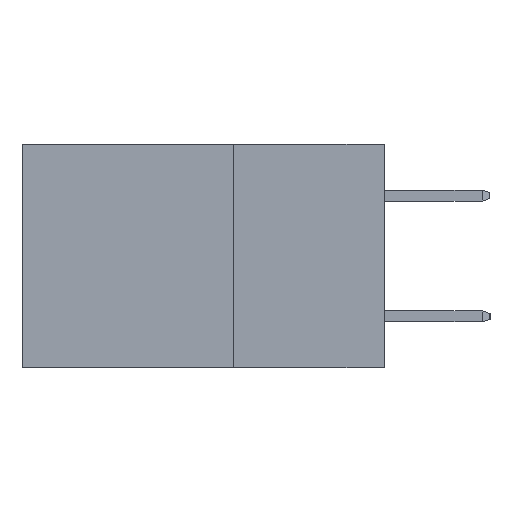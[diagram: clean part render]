
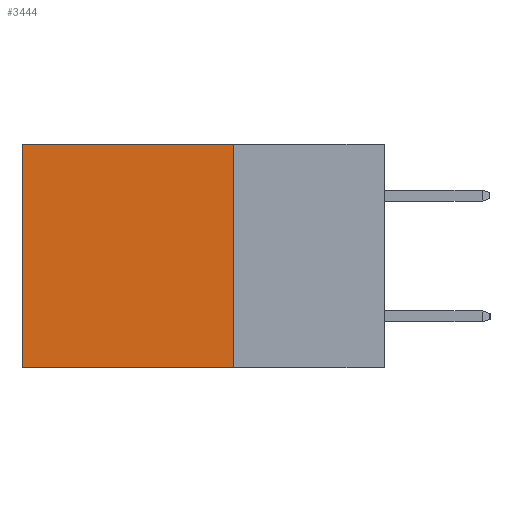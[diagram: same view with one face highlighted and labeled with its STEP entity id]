
A CAD part, left-side view. The second image highlights one B-rep face of the part: STEP entity #3444.
In plain terms, the highlighted planar face has unit normal (-1, 0, 0).
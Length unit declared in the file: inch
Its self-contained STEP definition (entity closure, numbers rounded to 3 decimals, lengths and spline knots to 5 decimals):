
#657 = CARTESIAN_POINT ( 'NONE',  ( 0.2615, 0.25, -0.37 ) ) ;
#1102 = ORIENTED_EDGE ( 'NONE', *, *, #1805, .T. ) ;
#1210 = EDGE_CURVE ( 'NONE', #1348, #4606, #9111, .T. ) ;
#1348 = VERTEX_POINT ( 'NONE', #11671 ) ;
#1699 = EDGE_CURVE ( 'NONE', #2932, #10370, #4565, .T. ) ;
#1805 = EDGE_CURVE ( 'NONE', #2932, #1348, #9880, .T. ) ;
#2069 = EDGE_CURVE ( 'NONE', #10370, #4606, #5583, .T. ) ;
#2316 = DIRECTION ( 'NONE',  ( 0., 0., -1. ) ) ;
#2762 = CARTESIAN_POINT ( 'NONE',  ( 0.2615, 0.25, -0.37 ) ) ;
#2932 = VERTEX_POINT ( 'NONE', #6329 ) ;
#3020 = ORIENTED_EDGE ( 'NONE', *, *, #2069, .F. ) ;
#3444 = ADVANCED_FACE ( 'NONE', ( #4428 ), #8945, .F. ) ;
#3583 = CARTESIAN_POINT ( 'NONE',  ( 0.2615, 0.25, -0.37 ) ) ;
#4061 = ORIENTED_EDGE ( 'NONE', *, *, #1210, .T. ) ;
#4428 = FACE_OUTER_BOUND ( 'NONE', #6059, .T. ) ;
#4563 = DIRECTION ( 'NONE',  ( 0., 0., -1. ) ) ;
#4565 = LINE ( 'NONE', #6421, #8715 ) ;
#4606 = VERTEX_POINT ( 'NONE', #6976 ) ;
#4660 = DIRECTION ( 'NONE',  ( 0., 1., 0. ) ) ;
#4981 = ORIENTED_EDGE ( 'NONE', *, *, #1699, .F. ) ;
#4996 = VECTOR ( 'NONE', #7368, 39.37008 ) ;
#5430 = CARTESIAN_POINT ( 'NONE',  ( 0.2615, 0.6, -0.37 ) ) ;
#5583 = LINE ( 'NONE', #3583, #9651 ) ;
#6059 = EDGE_LOOP ( 'NONE', ( #4061, #3020, #4981, #1102 ) ) ;
#6329 = CARTESIAN_POINT ( 'NONE',  ( 0.2615, 0.25, 0. ) ) ;
#6421 = CARTESIAN_POINT ( 'NONE',  ( 0.2615, 0.25, -0.37 ) ) ;
#6976 = CARTESIAN_POINT ( 'NONE',  ( 0.2615, 0.6, -0.37 ) ) ;
#7368 = DIRECTION ( 'NONE',  ( 0., 1., 0. ) ) ;
#8715 = VECTOR ( 'NONE', #10848, 39.37008 ) ;
#8945 = PLANE ( 'NONE',  #9903 ) ;
#9006 = CARTESIAN_POINT ( 'NONE',  ( 0.2615, 0.25, 0. ) ) ;
#9111 = LINE ( 'NONE', #5430, #10800 ) ;
#9651 = VECTOR ( 'NONE', #4660, 39.37008 ) ;
#9785 = DIRECTION ( 'NONE',  ( 1., 0., 0. ) ) ;
#9880 = LINE ( 'NONE', #9006, #4996 ) ;
#9903 = AXIS2_PLACEMENT_3D ( 'NONE', #657, #9785, #4563 ) ;
#10370 = VERTEX_POINT ( 'NONE', #2762 ) ;
#10800 = VECTOR ( 'NONE', #2316, 39.37008 ) ;
#10848 = DIRECTION ( 'NONE',  ( 0., 0., -1. ) ) ;
#11671 = CARTESIAN_POINT ( 'NONE',  ( 0.2615, 0.6, 0. ) ) ;
